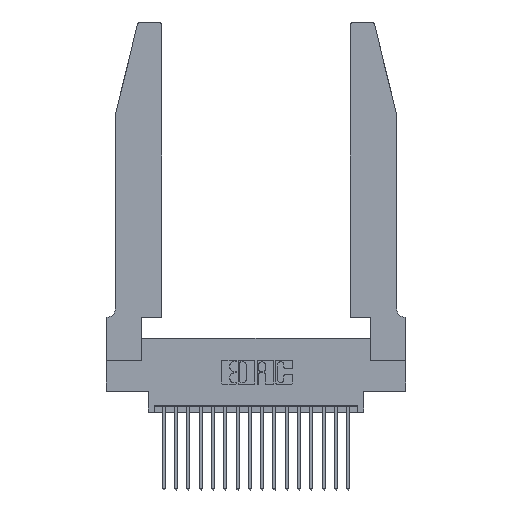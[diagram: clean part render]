
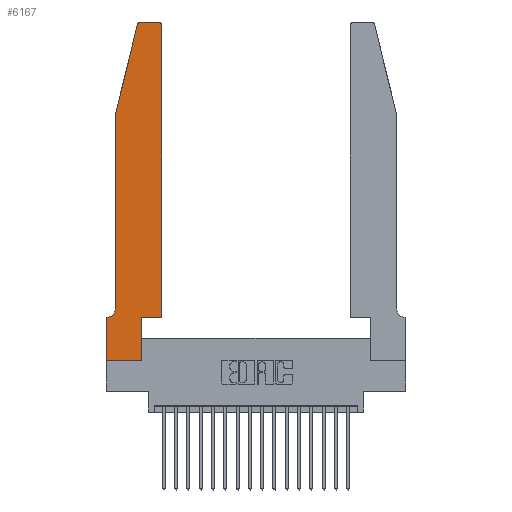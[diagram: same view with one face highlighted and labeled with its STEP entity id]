
A CAD part, top view. The second image highlights one B-rep face of the part: STEP entity #6167.
In plain terms, the highlighted planar face has unit normal (0, 0, 1).
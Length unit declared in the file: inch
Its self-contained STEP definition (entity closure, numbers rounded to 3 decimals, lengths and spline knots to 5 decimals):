
#171 = EDGE_CURVE ( 'NONE', #8229, #18835, #18228, .T. ) ;
#853 = CARTESIAN_POINT ( 'NONE',  ( 0.4205, 2.72, 0.37 ) ) ;
#1071 = DIRECTION ( 'NONE',  ( -0.239, -0.971, 0. ) ) ;
#1330 = CARTESIAN_POINT ( 'NONE',  ( 0., 0., 0.37 ) ) ;
#1420 = VECTOR ( 'NONE', #8054, 39.37008 ) ;
#1641 = ORIENTED_EDGE ( 'NONE', *, *, #14993, .T. ) ;
#2028 = LINE ( 'NONE', #16097, #14391 ) ;
#2048 = PLANE ( 'NONE',  #3301 ) ;
#2606 = DIRECTION ( 'NONE',  ( 1., 0., 0. ) ) ;
#2819 = ORIENTED_EDGE ( 'NONE', *, *, #18436, .T. ) ;
#3301 = AXIS2_PLACEMENT_3D ( 'NONE', #18191, #19777, #10374 ) ;
#3564 = VERTEX_POINT ( 'NONE', #16773 ) ;
#3627 = LINE ( 'NONE', #18140, #11180 ) ;
#3759 = VERTEX_POINT ( 'NONE', #4549 ) ;
#3911 = EDGE_CURVE ( 'NONE', #15716, #18111, #4207, .T. ) ;
#4207 = CIRCLE ( 'NONE', #20369, 0.07 ) ;
#4440 = ORIENTED_EDGE ( 'NONE', *, *, #19616, .T. ) ;
#4505 = EDGE_CURVE ( 'NONE', #3759, #6501, #2028, .T. ) ;
#4549 = CARTESIAN_POINT ( 'NONE',  ( 0.4505, 0.35, 0.37 ) ) ;
#4999 = FACE_OUTER_BOUND ( 'NONE', #10625, .T. ) ;
#5101 = CARTESIAN_POINT ( 'NONE',  ( 0.0755, 2., 0.37 ) ) ;
#5255 = DIRECTION ( 'NONE',  ( 1., 0., 0. ) ) ;
#5484 = EDGE_CURVE ( 'NONE', #3564, #8229, #3627, .T. ) ;
#5680 = VERTEX_POINT ( 'NONE', #12359 ) ;
#5831 = LINE ( 'NONE', #16740, #13712 ) ;
#6152 = ORIENTED_EDGE ( 'NONE', *, *, #20494, .T. ) ;
#6167 = ADVANCED_FACE ( 'NONE', ( #4999 ), #2048, .T. ) ;
#6426 = AXIS2_PLACEMENT_3D ( 'NONE', #19454, #16004, #5255 ) ;
#6434 = VECTOR ( 'NONE', #15411, 39.37008 ) ;
#6501 = VERTEX_POINT ( 'NONE', #15862 ) ;
#6780 = DIRECTION ( 'NONE',  ( 0., -1., 0. ) ) ;
#7036 = CARTESIAN_POINT ( 'NONE',  ( 0.0755, 2., 0.37 ) ) ;
#7136 = VERTEX_POINT ( 'NONE', #18922 ) ;
#7434 = ORIENTED_EDGE ( 'NONE', *, *, #11458, .T. ) ;
#7443 = LINE ( 'NONE', #20359, #10160 ) ;
#8054 = DIRECTION ( 'NONE',  ( 0., -1., 0. ) ) ;
#8195 = LINE ( 'NONE', #5101, #16012 ) ;
#8229 = VERTEX_POINT ( 'NONE', #12303 ) ;
#8274 = CARTESIAN_POINT ( 'NONE',  ( 0.0055, 0.42, 0.37 ) ) ;
#9077 = EDGE_CURVE ( 'NONE', #12969, #15716, #8195, .T. ) ;
#9792 = CARTESIAN_POINT ( 'NONE',  ( 0.0055, 0.35, 0.37 ) ) ;
#9849 = DIRECTION ( 'NONE',  ( -1., 0., 0. ) ) ;
#10130 = CARTESIAN_POINT ( 'NONE',  ( 0., 0., 0.37 ) ) ;
#10153 = CARTESIAN_POINT ( 'NONE',  ( 0., 0., 0.37 ) ) ;
#10160 = VECTOR ( 'NONE', #1071, 39.37008 ) ;
#10199 = LINE ( 'NONE', #1330, #1420 ) ;
#10374 = DIRECTION ( 'NONE',  ( 1., 0., 0. ) ) ;
#10401 = AXIS2_PLACEMENT_3D ( 'NONE', #853, #12296, #2606 ) ;
#10625 = EDGE_LOOP ( 'NONE', ( #20218, #11359, #6152, #10984, #11724, #16120, #1641, #4440, #12833, #7434, #16485, #2819 ) ) ;
#10984 = ORIENTED_EDGE ( 'NONE', *, *, #9077, .T. ) ;
#11180 = VECTOR ( 'NONE', #14971, 39.37008 ) ;
#11256 = CARTESIAN_POINT ( 'NONE',  ( 0.25487, 2.72718, 0.37 ) ) ;
#11359 = ORIENTED_EDGE ( 'NONE', *, *, #171, .T. ) ;
#11390 = VERTEX_POINT ( 'NONE', #20299 ) ;
#11458 = EDGE_CURVE ( 'NONE', #11390, #3759, #14744, .T. ) ;
#11710 = DIRECTION ( 'NONE',  ( 1., 0., 0. ) ) ;
#11724 = ORIENTED_EDGE ( 'NONE', *, *, #3911, .T. ) ;
#11955 = EDGE_CURVE ( 'NONE', #18111, #5680, #5831, .T. ) ;
#12296 = DIRECTION ( 'NONE',  ( 0., 0., 1. ) ) ;
#12303 = CARTESIAN_POINT ( 'NONE',  ( 0.284, 2.75, 0.37 ) ) ;
#12359 = CARTESIAN_POINT ( 'NONE',  ( 0., 0.35, 0.37 ) ) ;
#12581 = CARTESIAN_POINT ( 'NONE',  ( 0.4505, 0.35, 0.37 ) ) ;
#12833 = ORIENTED_EDGE ( 'NONE', *, *, #15826, .T. ) ;
#12969 = VERTEX_POINT ( 'NONE', #7036 ) ;
#13712 = VECTOR ( 'NONE', #15165, 39.37008 ) ;
#14130 = DIRECTION ( 'NONE',  ( 1., 0., 0. ) ) ;
#14224 = VECTOR ( 'NONE', #14130, 39.37008 ) ;
#14391 = VECTOR ( 'NONE', #16033, 39.37008 ) ;
#14744 = LINE ( 'NONE', #12581, #14224 ) ;
#14804 = LINE ( 'NONE', #17004, #6434 ) ;
#14971 = DIRECTION ( 'NONE',  ( -1., 0., 0. ) ) ;
#14993 = EDGE_CURVE ( 'NONE', #5680, #15219, #10199, .T. ) ;
#15154 = CARTESIAN_POINT ( 'NONE',  ( 0.0755, 0.42, 0.37 ) ) ;
#15165 = DIRECTION ( 'NONE',  ( -1., 0., 0. ) ) ;
#15219 = VERTEX_POINT ( 'NONE', #10130 ) ;
#15411 = DIRECTION ( 'NONE',  ( 0., 1., 0. ) ) ;
#15716 = VERTEX_POINT ( 'NONE', #15154 ) ;
#15826 = EDGE_CURVE ( 'NONE', #7136, #11390, #14804, .T. ) ;
#15862 = CARTESIAN_POINT ( 'NONE',  ( 0.4505, 2.72, 0.37 ) ) ;
#16004 = DIRECTION ( 'NONE',  ( 0., 0., 1. ) ) ;
#16012 = VECTOR ( 'NONE', #6780, 39.37008 ) ;
#16033 = DIRECTION ( 'NONE',  ( 0., 1., 0. ) ) ;
#16097 = CARTESIAN_POINT ( 'NONE',  ( 0.4505, 0.35, 0.37 ) ) ;
#16120 = ORIENTED_EDGE ( 'NONE', *, *, #11955, .T. ) ;
#16485 = ORIENTED_EDGE ( 'NONE', *, *, #4505, .T. ) ;
#16740 = CARTESIAN_POINT ( 'NONE',  ( 0.0755, 0.35, 0.37 ) ) ;
#16773 = CARTESIAN_POINT ( 'NONE',  ( 0.4205, 2.75, 0.37 ) ) ;
#17004 = CARTESIAN_POINT ( 'NONE',  ( 0.2865, 0.35, 0.37 ) ) ;
#17540 = LINE ( 'NONE', #10153, #20771 ) ;
#18111 = VERTEX_POINT ( 'NONE', #9792 ) ;
#18140 = CARTESIAN_POINT ( 'NONE',  ( 0.2605, 2.75, 0.37 ) ) ;
#18191 = CARTESIAN_POINT ( 'NONE',  ( 0., 0.35, 0.37 ) ) ;
#18228 = CIRCLE ( 'NONE', #6426, 0.03 ) ;
#18436 = EDGE_CURVE ( 'NONE', #6501, #3564, #20651, .T. ) ;
#18835 = VERTEX_POINT ( 'NONE', #11256 ) ;
#18922 = CARTESIAN_POINT ( 'NONE',  ( 0.2865, 0., 0.37 ) ) ;
#19270 = DIRECTION ( 'NONE',  ( 0., 0., -1. ) ) ;
#19454 = CARTESIAN_POINT ( 'NONE',  ( 0.284, 2.72, 0.37 ) ) ;
#19616 = EDGE_CURVE ( 'NONE', #15219, #7136, #17540, .T. ) ;
#19777 = DIRECTION ( 'NONE',  ( 0., 0., 1. ) ) ;
#20218 = ORIENTED_EDGE ( 'NONE', *, *, #5484, .T. ) ;
#20299 = CARTESIAN_POINT ( 'NONE',  ( 0.2865, 0.35, 0.37 ) ) ;
#20359 = CARTESIAN_POINT ( 'NONE',  ( 0.0755, 2., 0.37 ) ) ;
#20369 = AXIS2_PLACEMENT_3D ( 'NONE', #8274, #19270, #9849 ) ;
#20494 = EDGE_CURVE ( 'NONE', #18835, #12969, #7443, .T. ) ;
#20651 = CIRCLE ( 'NONE', #10401, 0.03 ) ;
#20771 = VECTOR ( 'NONE', #11710, 39.37008 ) ;
